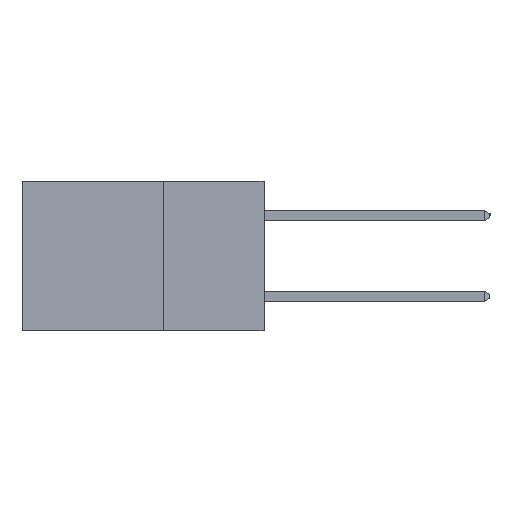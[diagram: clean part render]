
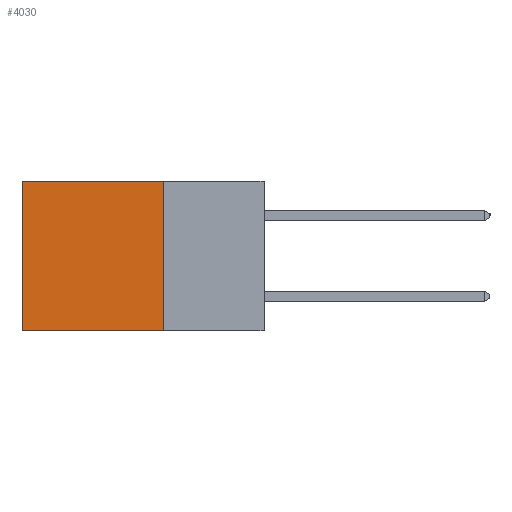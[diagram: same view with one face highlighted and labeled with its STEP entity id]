
A CAD part, left-side view. The second image highlights one B-rep face of the part: STEP entity #4030.
In plain terms, the highlighted planar face has unit normal (-1, 0, 0).
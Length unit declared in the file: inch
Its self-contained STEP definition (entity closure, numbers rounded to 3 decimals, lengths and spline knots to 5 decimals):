
#27 = VERTEX_POINT ( 'NONE', #4496 ) ;
#159 = VECTOR ( 'NONE', #2420, 39.37008 ) ;
#178 = DIRECTION ( 'NONE',  ( 0., 1., 0. ) ) ;
#565 = EDGE_CURVE ( 'NONE', #2871, #27, #6310, .T. ) ;
#605 = CARTESIAN_POINT ( 'NONE',  ( 0.2615, 0.6, -0.37 ) ) ;
#765 = CARTESIAN_POINT ( 'NONE',  ( 0.2615, 0.25, -0.37 ) ) ;
#781 = DIRECTION ( 'NONE',  ( 1., 0., 0. ) ) ;
#1247 = VERTEX_POINT ( 'NONE', #7741 ) ;
#1450 = EDGE_CURVE ( 'NONE', #1247, #11074, #3324, .T. ) ;
#1730 = ORIENTED_EDGE ( 'NONE', *, *, #4172, .F. ) ;
#1766 = PLANE ( 'NONE',  #5285 ) ;
#2420 = DIRECTION ( 'NONE',  ( 0., 1., 0. ) ) ;
#2871 = VERTEX_POINT ( 'NONE', #3023 ) ;
#3023 = CARTESIAN_POINT ( 'NONE',  ( 0.2615, 0.25, 0. ) ) ;
#3324 = LINE ( 'NONE', #9144, #159 ) ;
#3715 = CARTESIAN_POINT ( 'NONE',  ( 0.2615, 0.6, -0.37 ) ) ;
#4030 = ADVANCED_FACE ( 'NONE', ( #6150 ), #1766, .F. ) ;
#4042 = EDGE_LOOP ( 'NONE', ( #4810, #4951, #1730, #6378 ) ) ;
#4172 = EDGE_CURVE ( 'NONE', #2871, #1247, #5902, .T. ) ;
#4234 = VECTOR ( 'NONE', #8922, 39.37008 ) ;
#4322 = EDGE_CURVE ( 'NONE', #27, #11074, #4455, .T. ) ;
#4455 = LINE ( 'NONE', #3715, #4234 ) ;
#4496 = CARTESIAN_POINT ( 'NONE',  ( 0.2615, 0.6, 0. ) ) ;
#4810 = ORIENTED_EDGE ( 'NONE', *, *, #4322, .T. ) ;
#4951 = ORIENTED_EDGE ( 'NONE', *, *, #1450, .F. ) ;
#5226 = CARTESIAN_POINT ( 'NONE',  ( 0.2615, 0.25, 0. ) ) ;
#5285 = AXIS2_PLACEMENT_3D ( 'NONE', #8611, #781, #7759 ) ;
#5485 = VECTOR ( 'NONE', #8643, 39.37008 ) ;
#5902 = LINE ( 'NONE', #765, #5485 ) ;
#6150 = FACE_OUTER_BOUND ( 'NONE', #4042, .T. ) ;
#6310 = LINE ( 'NONE', #5226, #9151 ) ;
#6378 = ORIENTED_EDGE ( 'NONE', *, *, #565, .T. ) ;
#7741 = CARTESIAN_POINT ( 'NONE',  ( 0.2615, 0.25, -0.37 ) ) ;
#7759 = DIRECTION ( 'NONE',  ( 0., 0., -1. ) ) ;
#8611 = CARTESIAN_POINT ( 'NONE',  ( 0.2615, 0.25, -0.37 ) ) ;
#8643 = DIRECTION ( 'NONE',  ( 0., 0., -1. ) ) ;
#8922 = DIRECTION ( 'NONE',  ( 0., 0., -1. ) ) ;
#9144 = CARTESIAN_POINT ( 'NONE',  ( 0.2615, 0.25, -0.37 ) ) ;
#9151 = VECTOR ( 'NONE', #178, 39.37008 ) ;
#11074 = VERTEX_POINT ( 'NONE', #605 ) ;
